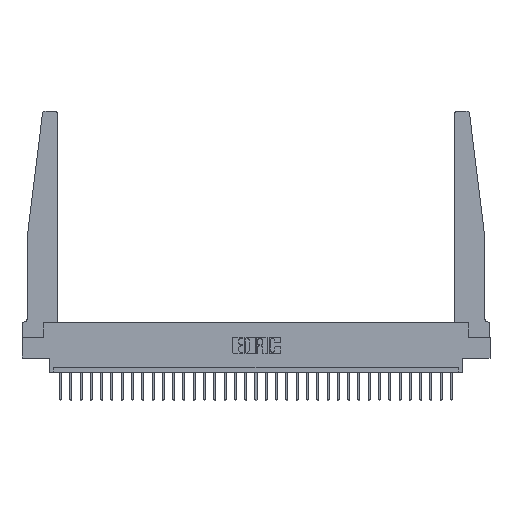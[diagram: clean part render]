
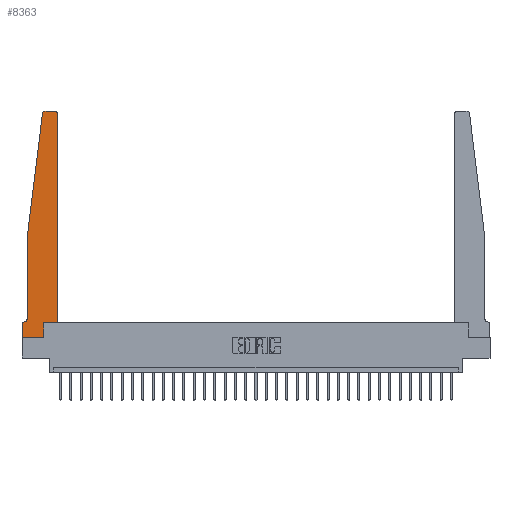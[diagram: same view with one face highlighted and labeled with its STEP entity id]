
A CAD part, top view. The second image highlights one B-rep face of the part: STEP entity #8363.
In plain terms, the highlighted planar face has unit normal (0, 0, 1).
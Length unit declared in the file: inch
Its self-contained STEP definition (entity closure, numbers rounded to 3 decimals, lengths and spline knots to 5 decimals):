
#289 = LINE ( 'NONE', #20974, #17810 ) ;
#1042 = LINE ( 'NONE', #14704, #7154 ) ;
#1293 = ORIENTED_EDGE ( 'NONE', *, *, #22408, .T. ) ;
#1993 = CARTESIAN_POINT ( 'NONE',  ( 0.395, 2.72, 0.37 ) ) ;
#2286 = VERTEX_POINT ( 'NONE', #23601 ) ;
#2322 = VERTEX_POINT ( 'NONE', #17524 ) ;
#2604 = VERTEX_POINT ( 'NONE', #10222 ) ;
#4213 = PLANE ( 'NONE',  #21788 ) ;
#4507 = DIRECTION ( 'NONE',  ( 1., 0., 0. ) ) ;
#4563 = EDGE_CURVE ( 'NONE', #2322, #16214, #24917, .T. ) ;
#4664 = EDGE_CURVE ( 'NONE', #7088, #16480, #289, .T. ) ;
#4768 = CARTESIAN_POINT ( 'NONE',  ( 0.065, 1.25, 0.37 ) ) ;
#5419 = ORIENTED_EDGE ( 'NONE', *, *, #17096, .T. ) ;
#5441 = ORIENTED_EDGE ( 'NONE', *, *, #18616, .T. ) ;
#5478 = EDGE_CURVE ( 'NONE', #22951, #14283, #14201, .T. ) ;
#5563 = EDGE_CURVE ( 'NONE', #2604, #25599, #16663, .T. ) ;
#5974 = VECTOR ( 'NONE', #20338, 39.37008 ) ;
#6402 = AXIS2_PLACEMENT_3D ( 'NONE', #22907, #27451, #29472 ) ;
#6550 = VERTEX_POINT ( 'NONE', #25864 ) ;
#6882 = ORIENTED_EDGE ( 'NONE', *, *, #16192, .T. ) ;
#7088 = VERTEX_POINT ( 'NONE', #23550 ) ;
#7154 = VECTOR ( 'NONE', #21451, 39.37008 ) ;
#7851 = DIRECTION ( 'NONE',  ( -1., 0., 0. ) ) ;
#8025 = AXIS2_PLACEMENT_3D ( 'NONE', #1993, #13593, #4507 ) ;
#8040 = ORIENTED_EDGE ( 'NONE', *, *, #20435, .T. ) ;
#8319 = VECTOR ( 'NONE', #11850, 39.37008 ) ;
#8363 = ADVANCED_FACE ( 'NONE', ( #19157 ), #4213, .T. ) ;
#9415 = VERTEX_POINT ( 'NONE', #17364 ) ;
#10222 = CARTESIAN_POINT ( 'NONE',  ( 0.24675, 2.72367, 0.37 ) ) ;
#10378 = CARTESIAN_POINT ( 'NONE',  ( 0.2605, 0., 0.37 ) ) ;
#10657 = EDGE_CURVE ( 'NONE', #25599, #2286, #15097, .T. ) ;
#10928 = EDGE_CURVE ( 'NONE', #16480, #2604, #23231, .T. ) ;
#11476 = CARTESIAN_POINT ( 'NONE',  ( 0., 0., 0.37 ) ) ;
#11586 = LINE ( 'NONE', #14979, #29019 ) ;
#11707 = DIRECTION ( 'NONE',  ( 0., 0., -1. ) ) ;
#11850 = DIRECTION ( 'NONE',  ( 0., -1., 0. ) ) ;
#12245 = DIRECTION ( 'NONE',  ( 0., 1., 0. ) ) ;
#12445 = CARTESIAN_POINT ( 'NONE',  ( 0.425, 0.18, 0.37 ) ) ;
#12787 = EDGE_CURVE ( 'NONE', #2286, #22951, #24562, .T. ) ;
#13593 = DIRECTION ( 'NONE',  ( 0., 0., 1. ) ) ;
#13900 = VECTOR ( 'NONE', #14665, 39.37008 ) ;
#13914 = CARTESIAN_POINT ( 'NONE',  ( 0.015, 0.2375, 0.37 ) ) ;
#14201 = LINE ( 'NONE', #24041, #24144 ) ;
#14283 = VERTEX_POINT ( 'NONE', #17115 ) ;
#14589 = VECTOR ( 'NONE', #12245, 39.37008 ) ;
#14665 = DIRECTION ( 'NONE',  ( 1., 0., 0. ) ) ;
#14704 = CARTESIAN_POINT ( 'NONE',  ( 0.425, 0.18, 0.37 ) ) ;
#14979 = CARTESIAN_POINT ( 'NONE',  ( 0., 0., 0.37 ) ) ;
#15012 = CARTESIAN_POINT ( 'NONE',  ( 0.425, 2.72, 0.37 ) ) ;
#15097 = LINE ( 'NONE', #25797, #8319 ) ;
#15686 = ORIENTED_EDGE ( 'NONE', *, *, #4563, .T. ) ;
#16116 = DIRECTION ( 'NONE',  ( -1., 0., 0. ) ) ;
#16192 = EDGE_CURVE ( 'NONE', #16214, #9415, #20106, .T. ) ;
#16214 = VERTEX_POINT ( 'NONE', #10378 ) ;
#16454 = DIRECTION ( 'NONE',  ( 0., 0., 1. ) ) ;
#16480 = VERTEX_POINT ( 'NONE', #17158 ) ;
#16575 = ORIENTED_EDGE ( 'NONE', *, *, #12787, .T. ) ;
#16663 = LINE ( 'NONE', #18344, #5974 ) ;
#17096 = EDGE_CURVE ( 'NONE', #26533, #7088, #17584, .T. ) ;
#17115 = CARTESIAN_POINT ( 'NONE',  ( 0., 0.1875, 0.37 ) ) ;
#17158 = CARTESIAN_POINT ( 'NONE',  ( 0.27653, 2.75, 0.37 ) ) ;
#17364 = CARTESIAN_POINT ( 'NONE',  ( 0.2605, 0.18, 0.37 ) ) ;
#17524 = CARTESIAN_POINT ( 'NONE',  ( 0., 0., 0.37 ) ) ;
#17584 = CIRCLE ( 'NONE', #8025, 0.03 ) ;
#17810 = VECTOR ( 'NONE', #7851, 39.37008 ) ;
#18344 = CARTESIAN_POINT ( 'NONE',  ( 0.065, 1.25, 0.37 ) ) ;
#18616 = EDGE_CURVE ( 'NONE', #9415, #6550, #1042, .T. ) ;
#19157 = FACE_OUTER_BOUND ( 'NONE', #26843, .T. ) ;
#19434 = CARTESIAN_POINT ( 'NONE',  ( 0.2605, 0.18, 0.37 ) ) ;
#19735 = DIRECTION ( 'NONE',  ( 0., -1., 0. ) ) ;
#20106 = LINE ( 'NONE', #19434, #27909 ) ;
#20144 = CARTESIAN_POINT ( 'NONE',  ( 0., 0.1875, 0.37 ) ) ;
#20338 = DIRECTION ( 'NONE',  ( -0.122, -0.992, 0. ) ) ;
#20435 = EDGE_CURVE ( 'NONE', #6550, #26533, #20617, .T. ) ;
#20617 = LINE ( 'NONE', #12445, #14589 ) ;
#20974 = CARTESIAN_POINT ( 'NONE',  ( 0.25, 2.75, 0.37 ) ) ;
#21451 = DIRECTION ( 'NONE',  ( 1., 0., 0. ) ) ;
#21788 = AXIS2_PLACEMENT_3D ( 'NONE', #20144, #16454, #23328 ) ;
#21810 = ORIENTED_EDGE ( 'NONE', *, *, #10928, .T. ) ;
#21921 = DIRECTION ( 'NONE',  ( 0., 1., 0. ) ) ;
#22389 = ORIENTED_EDGE ( 'NONE', *, *, #5478, .T. ) ;
#22408 = EDGE_CURVE ( 'NONE', #14283, #2322, #11586, .T. ) ;
#22903 = ORIENTED_EDGE ( 'NONE', *, *, #5563, .T. ) ;
#22907 = CARTESIAN_POINT ( 'NONE',  ( 0.27653, 2.72, 0.37 ) ) ;
#22951 = VERTEX_POINT ( 'NONE', #26379 ) ;
#23231 = CIRCLE ( 'NONE', #6402, 0.03 ) ;
#23328 = DIRECTION ( 'NONE',  ( 1., 0., 0. ) ) ;
#23550 = CARTESIAN_POINT ( 'NONE',  ( 0.395, 2.75, 0.37 ) ) ;
#23601 = CARTESIAN_POINT ( 'NONE',  ( 0.065, 0.2375, 0.37 ) ) ;
#24041 = CARTESIAN_POINT ( 'NONE',  ( 0.065, 0.1875, 0.37 ) ) ;
#24130 = DIRECTION ( 'NONE',  ( -1., 0., 0. ) ) ;
#24144 = VECTOR ( 'NONE', #24130, 39.37008 ) ;
#24529 = AXIS2_PLACEMENT_3D ( 'NONE', #13914, #11707, #16116 ) ;
#24562 = CIRCLE ( 'NONE', #24529, 0.05 ) ;
#24917 = LINE ( 'NONE', #11476, #13900 ) ;
#25599 = VERTEX_POINT ( 'NONE', #4768 ) ;
#25774 = ORIENTED_EDGE ( 'NONE', *, *, #4664, .T. ) ;
#25797 = CARTESIAN_POINT ( 'NONE',  ( 0.065, 1.25, 0.37 ) ) ;
#25864 = CARTESIAN_POINT ( 'NONE',  ( 0.425, 0.18, 0.37 ) ) ;
#26379 = CARTESIAN_POINT ( 'NONE',  ( 0.015, 0.1875, 0.37 ) ) ;
#26533 = VERTEX_POINT ( 'NONE', #15012 ) ;
#26644 = ORIENTED_EDGE ( 'NONE', *, *, #10657, .T. ) ;
#26843 = EDGE_LOOP ( 'NONE', ( #25774, #21810, #22903, #26644, #16575, #22389, #1293, #15686, #6882, #5441, #8040, #5419 ) ) ;
#27451 = DIRECTION ( 'NONE',  ( 0., 0., 1. ) ) ;
#27909 = VECTOR ( 'NONE', #21921, 39.37008 ) ;
#29019 = VECTOR ( 'NONE', #19735, 39.37008 ) ;
#29472 = DIRECTION ( 'NONE',  ( 1., 0., 0. ) ) ;
